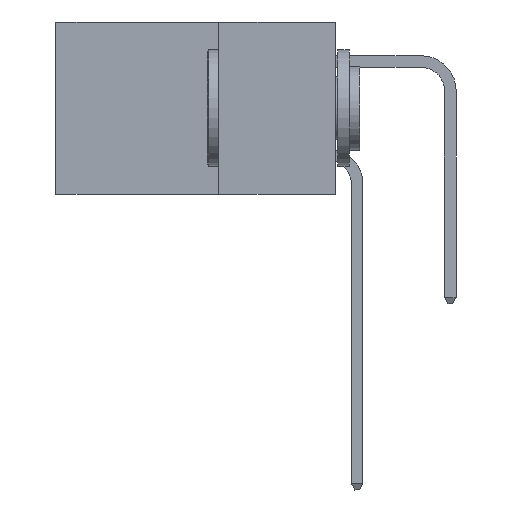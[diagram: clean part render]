
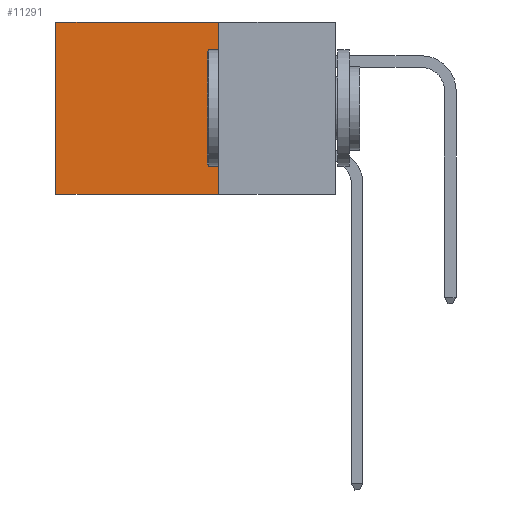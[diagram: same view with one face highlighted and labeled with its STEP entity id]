
A CAD part, left-side view. The second image highlights one B-rep face of the part: STEP entity #11291.
In plain terms, the highlighted planar face has unit normal (-1, 0, 0).
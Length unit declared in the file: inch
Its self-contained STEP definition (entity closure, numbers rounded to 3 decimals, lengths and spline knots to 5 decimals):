
#335 = AXIS2_PLACEMENT_3D ( 'NONE', #20331, #23389, #4888 ) ;
#831 = EDGE_CURVE ( 'NONE', #29875, #30236, #24806, .T. ) ;
#1946 = DIRECTION ( 'NONE',  ( 0., 0., -1. ) ) ;
#2242 = CARTESIAN_POINT ( 'NONE',  ( 0.2875, 0.25, 0. ) ) ;
#2729 = DIRECTION ( 'NONE',  ( 0., 0., -1. ) ) ;
#3606 = CARTESIAN_POINT ( 'NONE',  ( 0.2875, 0.6, -0.37 ) ) ;
#4888 = DIRECTION ( 'NONE',  ( 0., 0., -1. ) ) ;
#5176 = VECTOR ( 'NONE', #23289, 39.37008 ) ;
#8136 = CARTESIAN_POINT ( 'NONE',  ( 0.2875, 0.6, 0. ) ) ;
#8908 = LINE ( 'NONE', #22821, #33410 ) ;
#10952 = ORIENTED_EDGE ( 'NONE', *, *, #18747, .F. ) ;
#11291 = ADVANCED_FACE ( 'NONE', ( #38861 ), #38565, .F. ) ;
#15100 = EDGE_CURVE ( 'NONE', #31110, #29875, #8908, .T. ) ;
#15247 = EDGE_CURVE ( 'NONE', #31110, #39625, #26743, .T. ) ;
#15664 = VECTOR ( 'NONE', #2729, 39.37008 ) ;
#18747 = EDGE_CURVE ( 'NONE', #39625, #30236, #37840, .T. ) ;
#20331 = CARTESIAN_POINT ( 'NONE',  ( 0.2875, 0.25, 0. ) ) ;
#22821 = CARTESIAN_POINT ( 'NONE',  ( 0.2875, 0.25, 0. ) ) ;
#23289 = DIRECTION ( 'NONE',  ( 0., 1., 0. ) ) ;
#23389 = DIRECTION ( 'NONE',  ( 1., 0., 0. ) ) ;
#24410 = CARTESIAN_POINT ( 'NONE',  ( 0.2875, 0.6, 0. ) ) ;
#24806 = LINE ( 'NONE', #24410, #15664 ) ;
#25335 = EDGE_LOOP ( 'NONE', ( #33650, #10952, #31742, #29322 ) ) ;
#26743 = LINE ( 'NONE', #32698, #33859 ) ;
#28996 = DIRECTION ( 'NONE',  ( 0., 1., 0. ) ) ;
#29322 = ORIENTED_EDGE ( 'NONE', *, *, #15100, .T. ) ;
#29875 = VERTEX_POINT ( 'NONE', #8136 ) ;
#30236 = VERTEX_POINT ( 'NONE', #3606 ) ;
#31110 = VERTEX_POINT ( 'NONE', #2242 ) ;
#31742 = ORIENTED_EDGE ( 'NONE', *, *, #15247, .F. ) ;
#32698 = CARTESIAN_POINT ( 'NONE',  ( 0.2875, 0.25, 0. ) ) ;
#33410 = VECTOR ( 'NONE', #28996, 39.37008 ) ;
#33650 = ORIENTED_EDGE ( 'NONE', *, *, #831, .T. ) ;
#33859 = VECTOR ( 'NONE', #1946, 39.37008 ) ;
#35441 = CARTESIAN_POINT ( 'NONE',  ( 0.2875, 0.25, -0.37 ) ) ;
#37840 = LINE ( 'NONE', #35441, #5176 ) ;
#38565 = PLANE ( 'NONE',  #335 ) ;
#38861 = FACE_OUTER_BOUND ( 'NONE', #25335, .T. ) ;
#39234 = CARTESIAN_POINT ( 'NONE',  ( 0.2875, 0.25, -0.37 ) ) ;
#39625 = VERTEX_POINT ( 'NONE', #39234 ) ;
